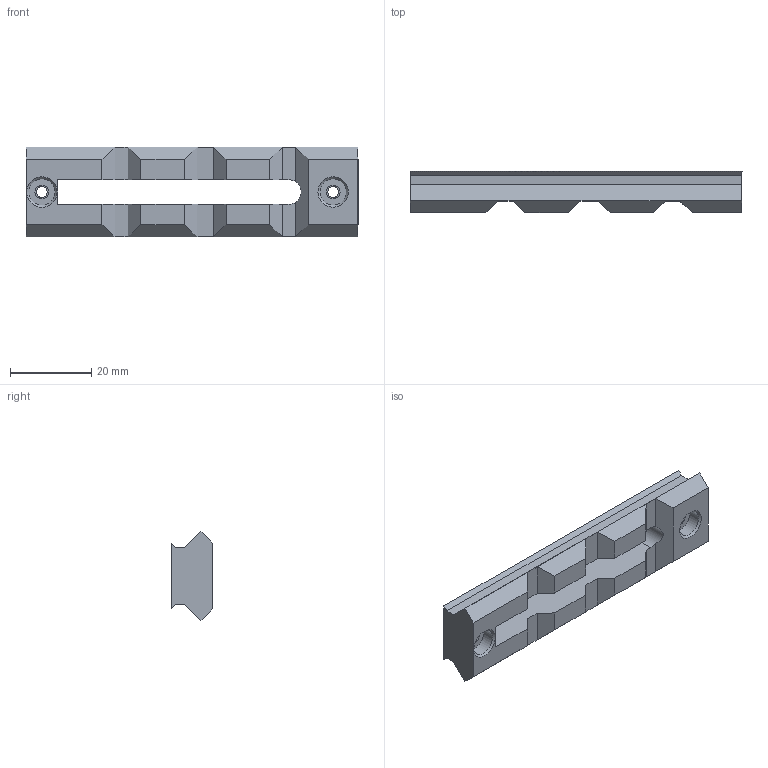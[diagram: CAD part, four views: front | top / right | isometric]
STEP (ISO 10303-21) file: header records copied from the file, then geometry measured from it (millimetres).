
FILE_DESCRIPTION (( 'STEP AP203' ), '1' );
FILE_NAME ('bottom_rail.STEP', '2020-05-10T06:01:17', ( '' ), ( '' ), 'SwSTEP 2.0', 'SolidWorks 2016', '' );
FILE_SCHEMA (( 'CONFIG_CONTROL_DESIGN' ));
Length unit declared in the file: millimetre
Products named in the file (1): bottom_rail
Bounding box: 81.81 x 10.28 x 22.05 mm (x, y, z)
Volume: 9710.5 mm3; surface area: 6011.1 mm2
Topology: 1 solids, 1 shells, 56 faces, 141 edges, 90 vertices
Faces by surface type: plane 47, cylinder 7, cone 2
Full cylindrical faces by diameter (mm): 2.7 x2, 3.4 x2, 6.5 x2
Entity records: 1677 total; most frequent: CARTESIAN_POINT 279, ORIENTED_EDGE 262, DIRECTION 261, EDGE_CURVE 131, VECTOR 113, LINE 113, VERTEX_POINT 88, AXIS2_PLACEMENT_3D 74
